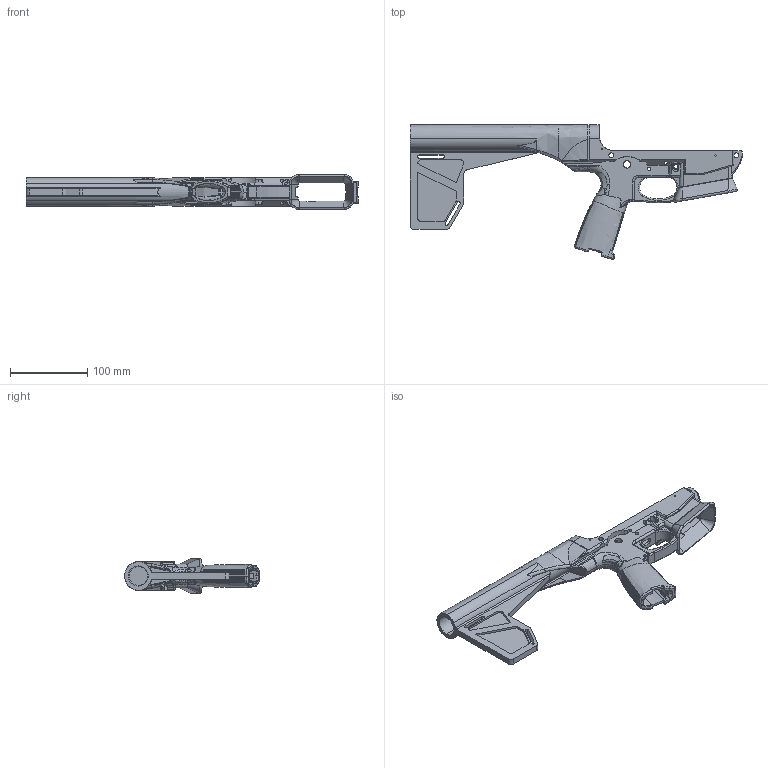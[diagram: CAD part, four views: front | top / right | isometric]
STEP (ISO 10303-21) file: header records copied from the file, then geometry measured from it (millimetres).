
FILE_DESCRIPTION (( 'STEP AP203' ), '1' );
FILE_NAME ('mbbi_monopoly_full_brace_v1.0.STEP', '2022-06-11T19:49:59', ( '' ), ( '' ), 'SwSTEP 2.0', 'SolidWorks 2021', '' );
FILE_SCHEMA (( 'CONFIG_CONTROL_DESIGN' ));
Products named in the file (1): mbbi_monopoly_full_brace_v1.0
Bounding box: 430.43 x 174.49 x 45.01 mm (x, y, z)
Volume: 393435.9 mm3; surface area: 149383.7 mm2
Topology: 1 solids, 3 shells, 1319 faces, 3788 edges, 2453 vertices
Faces by surface type: plane 517, bspline 387, cylinder 333, torus 52, sphere 22, cone 8
Entity records: 89750 total; most frequent: CARTESIAN_POINT 59411, ORIENTED_EDGE 7528, DIRECTION 4633, EDGE_CURVE 3764, VERTEX_POINT 2451, AXIS2_PLACEMENT_3D 1669, B_SPLINE_CURVE_WITH_KNOTS 1626, EDGE_LOOP 1363
